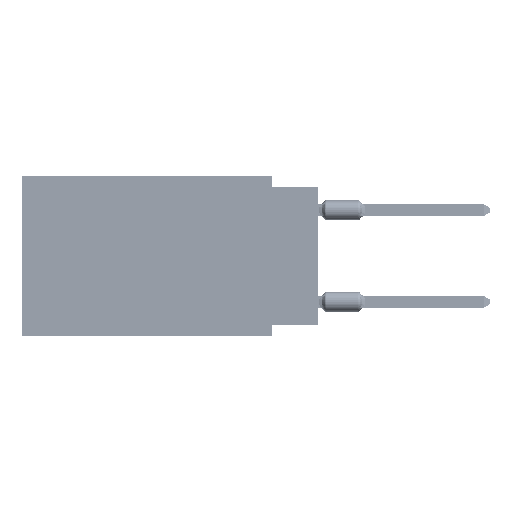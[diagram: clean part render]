
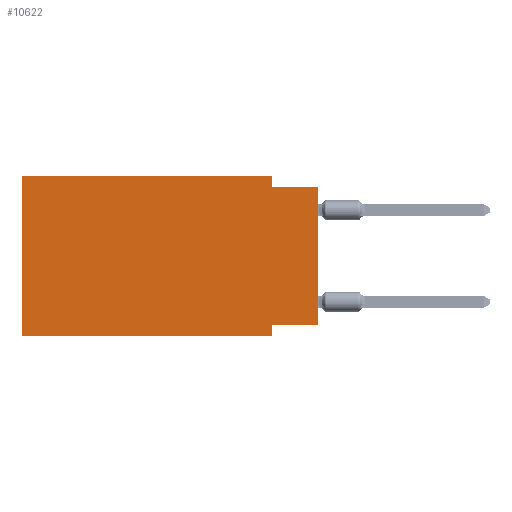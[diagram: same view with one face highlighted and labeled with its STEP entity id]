
A CAD part, left-side view. The second image highlights one B-rep face of the part: STEP entity #10622.
In plain terms, the highlighted planar face has unit normal (-1, 0, 0).
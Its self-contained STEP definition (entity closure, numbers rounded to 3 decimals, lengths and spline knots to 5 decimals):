
#1934 = CARTESIAN_POINT ( 'NONE',  ( 0., 0.1, -0.025 ) ) ;
#4006 = VECTOR ( 'NONE', #26364, 39.37008 ) ;
#5367 = ORIENTED_EDGE ( 'NONE', *, *, #53533, .F. ) ;
#5611 = DIRECTION ( 'NONE',  ( 0., 0., 1. ) ) ;
#5679 = EDGE_CURVE ( 'NONE', #51001, #63206, #41229, .T. ) ;
#10622 = ADVANCED_FACE ( 'NONE', ( #24463 ), #42048, .F. ) ;
#12713 = LINE ( 'NONE', #38360, #20109 ) ;
#13202 = VERTEX_POINT ( 'NONE', #1934 ) ;
#13306 = VECTOR ( 'NONE', #55867, 39.37008 ) ;
#14475 = LINE ( 'NONE', #34972, #43382 ) ;
#16442 = CARTESIAN_POINT ( 'NONE',  ( 0., 0., -0.025 ) ) ;
#16793 = VERTEX_POINT ( 'NONE', #16442 ) ;
#17950 = CARTESIAN_POINT ( 'NONE',  ( 0., 0.645, 0. ) ) ;
#18030 = VECTOR ( 'NONE', #60932, 39.37008 ) ;
#18381 = VERTEX_POINT ( 'NONE', #62163 ) ;
#18670 = ORIENTED_EDGE ( 'NONE', *, *, #24421, .F. ) ;
#18745 = ORIENTED_EDGE ( 'NONE', *, *, #47984, .F. ) ;
#19031 = EDGE_CURVE ( 'NONE', #67404, #16793, #14475, .T. ) ;
#19937 = EDGE_LOOP ( 'NONE', ( #50505, #55057, #49222, #5367, #18745, #63025, #66915, #18670 ) ) ;
#20109 = VECTOR ( 'NONE', #37935, 39.37008 ) ;
#22298 = EDGE_CURVE ( 'NONE', #13202, #16793, #56008, .T. ) ;
#22308 = CARTESIAN_POINT ( 'NONE',  ( 0., 0.1, -0.35 ) ) ;
#22727 = VERTEX_POINT ( 'NONE', #62740 ) ;
#22925 = CARTESIAN_POINT ( 'NONE',  ( 0., 0.645, -0.35 ) ) ;
#24421 = EDGE_CURVE ( 'NONE', #67404, #51001, #78003, .T. ) ;
#24463 = FACE_OUTER_BOUND ( 'NONE', #19937, .T. ) ;
#25349 = CARTESIAN_POINT ( 'NONE',  ( 0., 0., -0.325 ) ) ;
#26236 = CARTESIAN_POINT ( 'NONE',  ( 0., 0., -0.325 ) ) ;
#26364 = DIRECTION ( 'NONE',  ( 0., 0., -1. ) ) ;
#29078 = DIRECTION ( 'NONE',  ( 0., -1., 0. ) ) ;
#34812 = CARTESIAN_POINT ( 'NONE',  ( 0., 0.1, -0.35 ) ) ;
#34972 = CARTESIAN_POINT ( 'NONE',  ( 0., 0., 0. ) ) ;
#37935 = DIRECTION ( 'NONE',  ( 0., -1., 0. ) ) ;
#38360 = CARTESIAN_POINT ( 'NONE',  ( 0., 0.645, 0. ) ) ;
#39542 = VECTOR ( 'NONE', #29078, 39.37008 ) ;
#41229 = LINE ( 'NONE', #34812, #18030 ) ;
#42048 = PLANE ( 'NONE',  #69365 ) ;
#43018 = LINE ( 'NONE', #22925, #13306 ) ;
#43382 = VECTOR ( 'NONE', #54686, 39.37008 ) ;
#45220 = VECTOR ( 'NONE', #77565, 39.37008 ) ;
#47984 = EDGE_CURVE ( 'NONE', #18381, #63276, #52680, .T. ) ;
#49222 = ORIENTED_EDGE ( 'NONE', *, *, #64806, .F. ) ;
#50505 = ORIENTED_EDGE ( 'NONE', *, *, #19031, .T. ) ;
#51001 = VERTEX_POINT ( 'NONE', #67989 ) ;
#51812 = CARTESIAN_POINT ( 'NONE',  ( 0., 0.645, 0. ) ) ;
#52680 = LINE ( 'NONE', #51812, #74393 ) ;
#53533 = EDGE_CURVE ( 'NONE', #63276, #22727, #12713, .T. ) ;
#54686 = DIRECTION ( 'NONE',  ( 0., 0., 1. ) ) ;
#55057 = ORIENTED_EDGE ( 'NONE', *, *, #22298, .F. ) ;
#55867 = DIRECTION ( 'NONE',  ( 0., -1., 0. ) ) ;
#56008 = LINE ( 'NONE', #75280, #39542 ) ;
#58692 = CARTESIAN_POINT ( 'NONE',  ( 0., 0.645, 0. ) ) ;
#58887 = LINE ( 'NONE', #72156, #4006 ) ;
#60932 = DIRECTION ( 'NONE',  ( 0., 0., -1. ) ) ;
#62163 = CARTESIAN_POINT ( 'NONE',  ( 0., 0.645, -0.35 ) ) ;
#62740 = CARTESIAN_POINT ( 'NONE',  ( 0., 0.1, 0. ) ) ;
#63025 = ORIENTED_EDGE ( 'NONE', *, *, #74937, .T. ) ;
#63206 = VERTEX_POINT ( 'NONE', #22308 ) ;
#63276 = VERTEX_POINT ( 'NONE', #17950 ) ;
#64806 = EDGE_CURVE ( 'NONE', #22727, #13202, #58887, .T. ) ;
#66915 = ORIENTED_EDGE ( 'NONE', *, *, #5679, .F. ) ;
#67404 = VERTEX_POINT ( 'NONE', #26236 ) ;
#67989 = CARTESIAN_POINT ( 'NONE',  ( 0., 0.1, -0.325 ) ) ;
#69365 = AXIS2_PLACEMENT_3D ( 'NONE', #58692, #84399, #71548 ) ;
#71548 = DIRECTION ( 'NONE',  ( 0., 0., -1. ) ) ;
#72156 = CARTESIAN_POINT ( 'NONE',  ( 0., 0.1, 0. ) ) ;
#74393 = VECTOR ( 'NONE', #5611, 39.37008 ) ;
#74937 = EDGE_CURVE ( 'NONE', #18381, #63206, #43018, .T. ) ;
#75280 = CARTESIAN_POINT ( 'NONE',  ( 0., 0., -0.025 ) ) ;
#77565 = DIRECTION ( 'NONE',  ( 0., 1., 0. ) ) ;
#78003 = LINE ( 'NONE', #25349, #45220 ) ;
#84399 = DIRECTION ( 'NONE',  ( 1., 0., 0. ) ) ;
